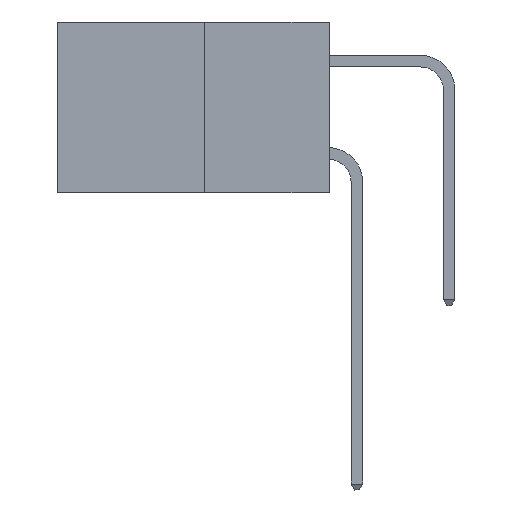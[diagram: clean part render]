
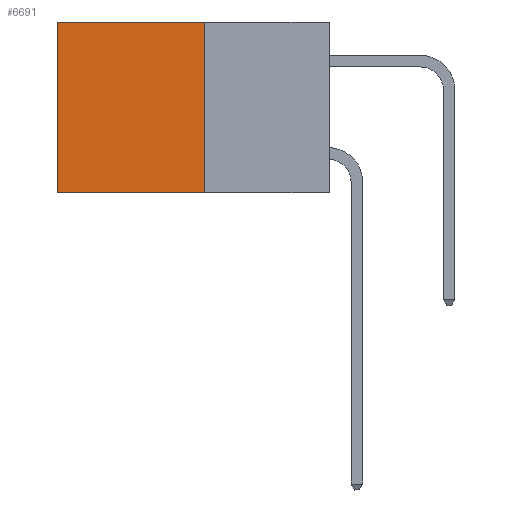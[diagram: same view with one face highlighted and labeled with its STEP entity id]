
A CAD part, left-side view. The second image highlights one B-rep face of the part: STEP entity #6691.
In plain terms, the highlighted planar face has unit normal (-1, 0, 0).
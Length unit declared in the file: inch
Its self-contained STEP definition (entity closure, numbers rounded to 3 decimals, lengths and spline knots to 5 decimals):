
#629 = VECTOR ( 'NONE', #10871, 39.37008 ) ;
#1344 = CARTESIAN_POINT ( 'NONE',  ( 0.277, 0.27, -0.37 ) ) ;
#1398 = EDGE_CURVE ( 'NONE', #11934, #24035, #9846, .T. ) ;
#1624 = FACE_OUTER_BOUND ( 'NONE', #11900, .T. ) ;
#3433 = CARTESIAN_POINT ( 'NONE',  ( 0.277, 0.27, -0.37 ) ) ;
#3889 = ORIENTED_EDGE ( 'NONE', *, *, #9164, .T. ) ;
#5744 = PLANE ( 'NONE',  #19985 ) ;
#6208 = VECTOR ( 'NONE', #16504, 39.37008 ) ;
#6691 = ADVANCED_FACE ( 'NONE', ( #1624 ), #5744, .F. ) ;
#7625 = DIRECTION ( 'NONE',  ( 1., 0., 0. ) ) ;
#9164 = EDGE_CURVE ( 'NONE', #22159, #11934, #15672, .T. ) ;
#9846 = LINE ( 'NONE', #13049, #23538 ) ;
#10358 = CARTESIAN_POINT ( 'NONE',  ( 0.277, 0.59, 0. ) ) ;
#10871 = DIRECTION ( 'NONE',  ( 0., 1., 0. ) ) ;
#10891 = ORIENTED_EDGE ( 'NONE', *, *, #14973, .F. ) ;
#11900 = EDGE_LOOP ( 'NONE', ( #18549, #13761, #10891, #3889 ) ) ;
#11934 = VERTEX_POINT ( 'NONE', #10358 ) ;
#12278 = DIRECTION ( 'NONE',  ( 0., 1., 0. ) ) ;
#12413 = DIRECTION ( 'NONE',  ( 0., 0., -1. ) ) ;
#12548 = CARTESIAN_POINT ( 'NONE',  ( 0.277, 0.27, 0. ) ) ;
#13049 = CARTESIAN_POINT ( 'NONE',  ( 0.277, 0.59, -0.37 ) ) ;
#13761 = ORIENTED_EDGE ( 'NONE', *, *, #23365, .F. ) ;
#13866 = CARTESIAN_POINT ( 'NONE',  ( 0.277, 0.59, -0.37 ) ) ;
#14007 = VERTEX_POINT ( 'NONE', #1344 ) ;
#14573 = LINE ( 'NONE', #16034, #19522 ) ;
#14973 = EDGE_CURVE ( 'NONE', #22159, #14007, #16198, .T. ) ;
#15672 = LINE ( 'NONE', #16553, #629 ) ;
#16034 = CARTESIAN_POINT ( 'NONE',  ( 0.277, 0.27, -0.37 ) ) ;
#16198 = LINE ( 'NONE', #3433, #6208 ) ;
#16504 = DIRECTION ( 'NONE',  ( 0., 0., -1. ) ) ;
#16553 = CARTESIAN_POINT ( 'NONE',  ( 0.277, 0.27, 0. ) ) ;
#18549 = ORIENTED_EDGE ( 'NONE', *, *, #1398, .T. ) ;
#19522 = VECTOR ( 'NONE', #12278, 39.37008 ) ;
#19985 = AXIS2_PLACEMENT_3D ( 'NONE', #22413, #7625, #20714 ) ;
#20714 = DIRECTION ( 'NONE',  ( 0., 0., -1. ) ) ;
#22159 = VERTEX_POINT ( 'NONE', #12548 ) ;
#22413 = CARTESIAN_POINT ( 'NONE',  ( 0.277, 0.27, -0.37 ) ) ;
#23365 = EDGE_CURVE ( 'NONE', #14007, #24035, #14573, .T. ) ;
#23538 = VECTOR ( 'NONE', #12413, 39.37008 ) ;
#24035 = VERTEX_POINT ( 'NONE', #13866 ) ;
